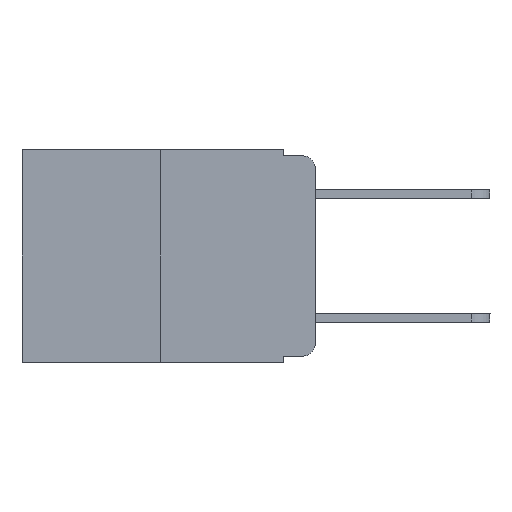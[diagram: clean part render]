
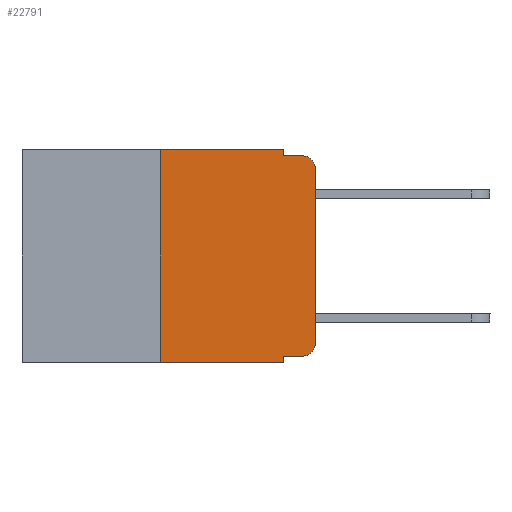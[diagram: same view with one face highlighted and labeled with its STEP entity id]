
A CAD part, left-side view. The second image highlights one B-rep face of the part: STEP entity #22791.
In plain terms, the highlighted planar face has unit normal (-1, 0, 0).
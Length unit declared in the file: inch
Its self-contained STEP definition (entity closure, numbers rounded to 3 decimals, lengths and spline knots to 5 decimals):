
#478 = CARTESIAN_POINT ( 'NONE',  ( 0., 0.25, 0. ) ) ;
#1069 = FACE_OUTER_BOUND ( 'NONE', #6340, .T. ) ;
#1140 = VERTEX_POINT ( 'NONE', #478 ) ;
#1334 = CARTESIAN_POINT ( 'NONE',  ( 0., 0.473, 0. ) ) ;
#1535 = VERTEX_POINT ( 'NONE', #1598 ) ;
#1555 = DIRECTION ( 'NONE',  ( 0., -1., 0. ) ) ;
#1598 = CARTESIAN_POINT ( 'NONE',  ( 0., 0., -0.313 ) ) ;
#1632 = AXIS2_PLACEMENT_3D ( 'NONE', #5141, #10848, #8748 ) ;
#2365 = CIRCLE ( 'NONE', #11256, 0.02 ) ;
#2805 = VERTEX_POINT ( 'NONE', #18160 ) ;
#3892 = ORIENTED_EDGE ( 'NONE', *, *, #20137, .F. ) ;
#4145 = LINE ( 'NONE', #18993, #7369 ) ;
#4181 = ORIENTED_EDGE ( 'NONE', *, *, #14751, .T. ) ;
#4197 = CARTESIAN_POINT ( 'NONE',  ( 0., 0.051, -0.343 ) ) ;
#4226 = ORIENTED_EDGE ( 'NONE', *, *, #5666, .T. ) ;
#5001 = CARTESIAN_POINT ( 'NONE',  ( 0., 0.051, -0.333 ) ) ;
#5141 = CARTESIAN_POINT ( 'NONE',  ( 0., 0.473, 0. ) ) ;
#5157 = VERTEX_POINT ( 'NONE', #18665 ) ;
#5253 = AXIS2_PLACEMENT_3D ( 'NONE', #20409, #16182, #16838 ) ;
#5666 = EDGE_CURVE ( 'NONE', #2805, #6435, #21113, .T. ) ;
#5706 = CARTESIAN_POINT ( 'NONE',  ( 0., 0.051, 0. ) ) ;
#5861 = VERTEX_POINT ( 'NONE', #16461 ) ;
#5947 = CIRCLE ( 'NONE', #5253, 0.02 ) ;
#6340 = EDGE_LOOP ( 'NONE', ( #4181, #23933, #11325, #11904, #9604, #18909, #4226, #3892, #23451, #21550 ) ) ;
#6435 = VERTEX_POINT ( 'NONE', #4197 ) ;
#6786 = CARTESIAN_POINT ( 'NONE',  ( 0., 0.051, -0.01 ) ) ;
#6961 = PLANE ( 'NONE',  #1632 ) ;
#7369 = VECTOR ( 'NONE', #11876, 39.37008 ) ;
#8292 = VERTEX_POINT ( 'NONE', #9436 ) ;
#8748 = DIRECTION ( 'NONE',  ( 0., 0., -1. ) ) ;
#8796 = DIRECTION ( 'NONE',  ( 0., -1., 0. ) ) ;
#8801 = DIRECTION ( 'NONE',  ( 0., 0., 1. ) ) ;
#8981 = CARTESIAN_POINT ( 'NONE',  ( 0., 0.051, -0.01 ) ) ;
#9133 = CARTESIAN_POINT ( 'NONE',  ( 0., 0.25, 0. ) ) ;
#9436 = CARTESIAN_POINT ( 'NONE',  ( 0., 0.051, -0.333 ) ) ;
#9604 = ORIENTED_EDGE ( 'NONE', *, *, #12992, .F. ) ;
#10417 = VECTOR ( 'NONE', #8801, 39.37008 ) ;
#10618 = EDGE_CURVE ( 'NONE', #2805, #1140, #10637, .T. ) ;
#10637 = LINE ( 'NONE', #9133, #11784 ) ;
#10848 = DIRECTION ( 'NONE',  ( 1., 0., 0. ) ) ;
#11058 = VECTOR ( 'NONE', #1555, 39.37008 ) ;
#11256 = AXIS2_PLACEMENT_3D ( 'NONE', #23660, #20510, #18655 ) ;
#11294 = VECTOR ( 'NONE', #11489, 39.37008 ) ;
#11325 = ORIENTED_EDGE ( 'NONE', *, *, #23121, .F. ) ;
#11489 = DIRECTION ( 'NONE',  ( 0., -1., 0. ) ) ;
#11784 = VECTOR ( 'NONE', #17024, 39.37008 ) ;
#11876 = DIRECTION ( 'NONE',  ( 0., 0., -1. ) ) ;
#11904 = ORIENTED_EDGE ( 'NONE', *, *, #11972, .F. ) ;
#11972 = EDGE_CURVE ( 'NONE', #5157, #20066, #4145, .T. ) ;
#12315 = LINE ( 'NONE', #5706, #21565 ) ;
#12959 = LINE ( 'NONE', #6786, #13542 ) ;
#12992 = EDGE_CURVE ( 'NONE', #1140, #5157, #14531, .T. ) ;
#13542 = VECTOR ( 'NONE', #21270, 39.37008 ) ;
#13594 = EDGE_CURVE ( 'NONE', #8292, #17513, #16538, .T. ) ;
#14531 = LINE ( 'NONE', #1334, #18291 ) ;
#14751 = EDGE_CURVE ( 'NONE', #1535, #20133, #15878, .T. ) ;
#15878 = LINE ( 'NONE', #16131, #10417 ) ;
#16131 = CARTESIAN_POINT ( 'NONE',  ( 0., 0., 0. ) ) ;
#16182 = DIRECTION ( 'NONE',  ( -1., 0., 0. ) ) ;
#16461 = CARTESIAN_POINT ( 'NONE',  ( 0., 0.02, -0.01 ) ) ;
#16538 = LINE ( 'NONE', #5001, #11058 ) ;
#16718 = CARTESIAN_POINT ( 'NONE',  ( 0., 0., -0.03 ) ) ;
#16838 = DIRECTION ( 'NONE',  ( 0., 0., -1. ) ) ;
#17024 = DIRECTION ( 'NONE',  ( 0., 0., 1. ) ) ;
#17513 = VERTEX_POINT ( 'NONE', #19930 ) ;
#18160 = CARTESIAN_POINT ( 'NONE',  ( 0., 0.25, -0.343 ) ) ;
#18291 = VECTOR ( 'NONE', #8796, 39.37008 ) ;
#18655 = DIRECTION ( 'NONE',  ( 0., 0., -1. ) ) ;
#18665 = CARTESIAN_POINT ( 'NONE',  ( 0., 0.051, 0. ) ) ;
#18680 = EDGE_CURVE ( 'NONE', #17513, #1535, #5947, .T. ) ;
#18909 = ORIENTED_EDGE ( 'NONE', *, *, #10618, .F. ) ;
#18993 = CARTESIAN_POINT ( 'NONE',  ( 0., 0.051, 0. ) ) ;
#19930 = CARTESIAN_POINT ( 'NONE',  ( 0., 0.02, -0.333 ) ) ;
#20066 = VERTEX_POINT ( 'NONE', #8981 ) ;
#20133 = VERTEX_POINT ( 'NONE', #16718 ) ;
#20137 = EDGE_CURVE ( 'NONE', #8292, #6435, #12315, .T. ) ;
#20280 = DIRECTION ( 'NONE',  ( 0., 0., -1. ) ) ;
#20409 = CARTESIAN_POINT ( 'NONE',  ( 0., 0.02, -0.313 ) ) ;
#20510 = DIRECTION ( 'NONE',  ( -1., 0., 0. ) ) ;
#20623 = CARTESIAN_POINT ( 'NONE',  ( 0., 0.473, -0.343 ) ) ;
#21113 = LINE ( 'NONE', #20623, #11294 ) ;
#21270 = DIRECTION ( 'NONE',  ( 0., -1., 0. ) ) ;
#21550 = ORIENTED_EDGE ( 'NONE', *, *, #18680, .T. ) ;
#21565 = VECTOR ( 'NONE', #20280, 39.37008 ) ;
#21686 = EDGE_CURVE ( 'NONE', #20133, #5861, #2365, .T. ) ;
#22791 = ADVANCED_FACE ( 'NONE', ( #1069 ), #6961, .F. ) ;
#23121 = EDGE_CURVE ( 'NONE', #20066, #5861, #12959, .T. ) ;
#23451 = ORIENTED_EDGE ( 'NONE', *, *, #13594, .T. ) ;
#23660 = CARTESIAN_POINT ( 'NONE',  ( 0., 0.02, -0.03 ) ) ;
#23933 = ORIENTED_EDGE ( 'NONE', *, *, #21686, .T. ) ;
